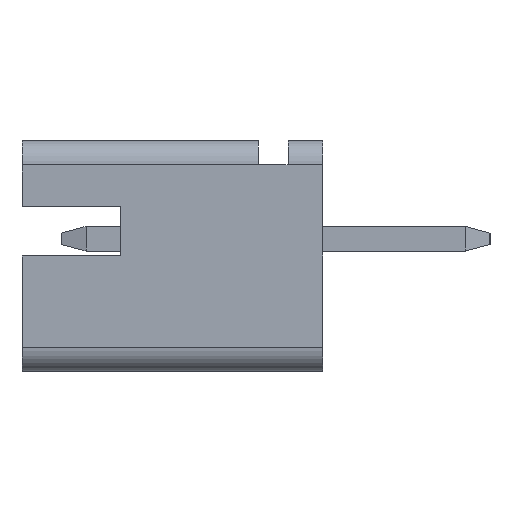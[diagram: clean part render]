
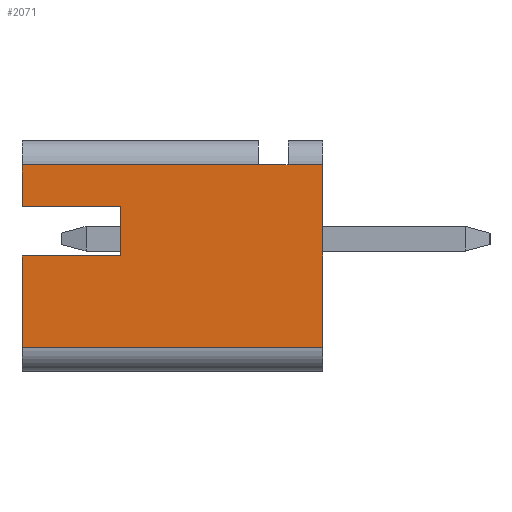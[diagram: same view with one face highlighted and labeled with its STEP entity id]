
A CAD part, left-side view. The second image highlights one B-rep face of the part: STEP entity #2071.
In plain terms, the highlighted planar face has unit normal (-1, 0, 0).
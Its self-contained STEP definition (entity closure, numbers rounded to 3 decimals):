
#89 = EDGE_CURVE ( 'NONE', #4544, #3480, #1114, .T. ) ;
#381 = CARTESIAN_POINT ( 'NONE',  ( -2., 6.1, 2. ) ) ;
#415 = ORIENTED_EDGE ( 'NONE', *, *, #2420, .T. ) ;
#599 = DIRECTION ( 'NONE',  ( 0., 0., 1. ) ) ;
#614 = CARTESIAN_POINT ( 'NONE',  ( -2., 6.1, -0.35 ) ) ;
#675 = EDGE_CURVE ( 'NONE', #5207, #744, #2501, .T. ) ;
#744 = VERTEX_POINT ( 'NONE', #4850 ) ;
#882 = EDGE_LOOP ( 'NONE', ( #4980, #2981, #3414, #415, #1261, #5369, #1159, #4585, #3372, #2263 ) ) ;
#944 = EDGE_CURVE ( 'NONE', #3949, #1564, #1997, .T. ) ;
#1114 = LINE ( 'NONE', #2482, #4257 ) ;
#1151 = VERTEX_POINT ( 'NONE', #5496 ) ;
#1159 = ORIENTED_EDGE ( 'NONE', *, *, #675, .F. ) ;
#1261 = ORIENTED_EDGE ( 'NONE', *, *, #89, .F. ) ;
#1344 = CARTESIAN_POINT ( 'NONE',  ( -2., 4.1, 0.65 ) ) ;
#1487 = CARTESIAN_POINT ( 'NONE',  ( -2., 0., -2.2 ) ) ;
#1516 = VECTOR ( 'NONE', #599, 1000. ) ;
#1518 = DIRECTION ( 'NONE',  ( 0., -1., 0. ) ) ;
#1564 = VERTEX_POINT ( 'NONE', #3856 ) ;
#1607 = VECTOR ( 'NONE', #1518, 1000. ) ;
#1676 = CARTESIAN_POINT ( 'NONE',  ( -2., 1.3, 1.5 ) ) ;
#1724 = FACE_OUTER_BOUND ( 'NONE', #882, .T. ) ;
#1743 = LINE ( 'NONE', #4664, #4149 ) ;
#1869 = CARTESIAN_POINT ( 'NONE',  ( -2., 6.1, -0.35 ) ) ;
#1997 = LINE ( 'NONE', #2839, #5346 ) ;
#2071 = ADVANCED_FACE ( 'NONE', ( #1724 ), #3431, .F. ) ;
#2087 = DIRECTION ( 'NONE',  ( 0., 0., 1. ) ) ;
#2142 = VERTEX_POINT ( 'NONE', #1869 ) ;
#2222 = EDGE_CURVE ( 'NONE', #4258, #5207, #2313, .T. ) ;
#2241 = VERTEX_POINT ( 'NONE', #3067 ) ;
#2263 = ORIENTED_EDGE ( 'NONE', *, *, #3043, .F. ) ;
#2313 = LINE ( 'NONE', #3607, #3259 ) ;
#2420 = EDGE_CURVE ( 'NONE', #3949, #3480, #1743, .T. ) ;
#2482 = CARTESIAN_POINT ( 'NONE',  ( -2., 1.3, 1.5 ) ) ;
#2501 = LINE ( 'NONE', #381, #4668 ) ;
#2597 = CARTESIAN_POINT ( 'NONE',  ( -2., 0.7, 1.5 ) ) ;
#2839 = CARTESIAN_POINT ( 'NONE',  ( -2., 0., 2. ) ) ;
#2941 = VECTOR ( 'NONE', #5186, 1000. ) ;
#2959 = DIRECTION ( 'NONE',  ( 1., 0., 0. ) ) ;
#2981 = ORIENTED_EDGE ( 'NONE', *, *, #3168, .T. ) ;
#2985 = CARTESIAN_POINT ( 'NONE',  ( -2., 0., 1.5 ) ) ;
#3043 = EDGE_CURVE ( 'NONE', #2142, #2241, #3055, .T. ) ;
#3055 = LINE ( 'NONE', #3927, #2941 ) ;
#3057 = EDGE_CURVE ( 'NONE', #2241, #4258, #3138, .T. ) ;
#3067 = CARTESIAN_POINT ( 'NONE',  ( -2., 4.1, -0.35 ) ) ;
#3138 = LINE ( 'NONE', #1344, #1516 ) ;
#3168 = EDGE_CURVE ( 'NONE', #1151, #1564, #5416, .T. ) ;
#3259 = VECTOR ( 'NONE', #5315, 1000. ) ;
#3313 = DIRECTION ( 'NONE',  ( 0., 0., 1. ) ) ;
#3372 = ORIENTED_EDGE ( 'NONE', *, *, #3057, .F. ) ;
#3379 = DIRECTION ( 'NONE',  ( 0., 0., -1. ) ) ;
#3414 = ORIENTED_EDGE ( 'NONE', *, *, #944, .F. ) ;
#3431 = PLANE ( 'NONE',  #3789 ) ;
#3480 = VERTEX_POINT ( 'NONE', #2597 ) ;
#3491 = CARTESIAN_POINT ( 'NONE',  ( -2., 0., 0. ) ) ;
#3607 = CARTESIAN_POINT ( 'NONE',  ( -2., 6.1, 0.65 ) ) ;
#3611 = VECTOR ( 'NONE', #3313, 1000. ) ;
#3725 = DIRECTION ( 'NONE',  ( 0., -1., 0. ) ) ;
#3789 = AXIS2_PLACEMENT_3D ( 'NONE', #3491, #2959, #3379 ) ;
#3856 = CARTESIAN_POINT ( 'NONE',  ( -2., 0., -2.2 ) ) ;
#3927 = CARTESIAN_POINT ( 'NONE',  ( -2., 6.1, -0.35 ) ) ;
#3930 = EDGE_CURVE ( 'NONE', #1151, #2142, #4150, .T. ) ;
#3949 = VERTEX_POINT ( 'NONE', #4185 ) ;
#3950 = CARTESIAN_POINT ( 'NONE',  ( -2., 4.1, 0.65 ) ) ;
#4149 = VECTOR ( 'NONE', #4321, 1000. ) ;
#4150 = LINE ( 'NONE', #614, #3611 ) ;
#4185 = CARTESIAN_POINT ( 'NONE',  ( -2., 0., 1.5 ) ) ;
#4186 = DIRECTION ( 'NONE',  ( 0., 0., -1. ) ) ;
#4257 = VECTOR ( 'NONE', #3725, 1000. ) ;
#4258 = VERTEX_POINT ( 'NONE', #3950 ) ;
#4321 = DIRECTION ( 'NONE',  ( 0., 1., 0. ) ) ;
#4544 = VERTEX_POINT ( 'NONE', #1676 ) ;
#4585 = ORIENTED_EDGE ( 'NONE', *, *, #2222, .F. ) ;
#4614 = LINE ( 'NONE', #2985, #5425 ) ;
#4664 = CARTESIAN_POINT ( 'NONE',  ( -2., 0., 1.5 ) ) ;
#4668 = VECTOR ( 'NONE', #2087, 1000. ) ;
#4850 = CARTESIAN_POINT ( 'NONE',  ( -2., 6.1, 1.5 ) ) ;
#4980 = ORIENTED_EDGE ( 'NONE', *, *, #3930, .F. ) ;
#4995 = EDGE_CURVE ( 'NONE', #4544, #744, #4614, .T. ) ;
#5186 = DIRECTION ( 'NONE',  ( 0., -1., 0. ) ) ;
#5207 = VERTEX_POINT ( 'NONE', #5259 ) ;
#5259 = CARTESIAN_POINT ( 'NONE',  ( -2., 6.1, 0.65 ) ) ;
#5315 = DIRECTION ( 'NONE',  ( 0., 1., 0. ) ) ;
#5346 = VECTOR ( 'NONE', #4186, 1000. ) ;
#5369 = ORIENTED_EDGE ( 'NONE', *, *, #4995, .T. ) ;
#5416 = LINE ( 'NONE', #1487, #1607 ) ;
#5425 = VECTOR ( 'NONE', #5486, 1000. ) ;
#5486 = DIRECTION ( 'NONE',  ( 0., 1., 0. ) ) ;
#5496 = CARTESIAN_POINT ( 'NONE',  ( -2., 6.1, -2.2 ) ) ;
